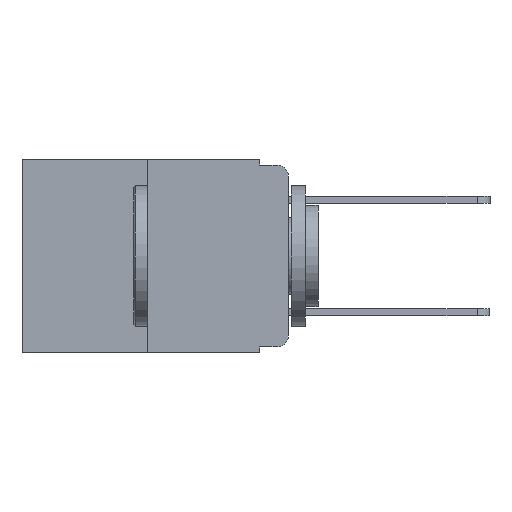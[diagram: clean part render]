
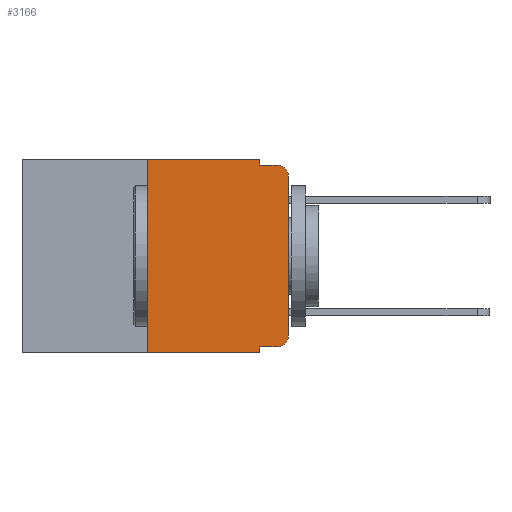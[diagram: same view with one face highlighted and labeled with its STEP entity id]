
A CAD part, left-side view. The second image highlights one B-rep face of the part: STEP entity #3166.
In plain terms, the highlighted planar face has unit normal (-1, 0, 0).
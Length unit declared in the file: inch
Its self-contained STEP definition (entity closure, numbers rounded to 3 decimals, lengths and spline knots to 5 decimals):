
#98 = CARTESIAN_POINT ( 'NONE',  ( 0., 0.25, 0. ) ) ;
#194 = CARTESIAN_POINT ( 'NONE',  ( 0., 0.02, -0.03 ) ) ;
#332 = LINE ( 'NONE', #822, #599 ) ;
#370 = VERTEX_POINT ( 'NONE', #8942 ) ;
#573 = EDGE_LOOP ( 'NONE', ( #9256, #2607, #1830, #5777, #4841, #9421, #8295, #3054, #5703, #5567 ) ) ;
#583 = CARTESIAN_POINT ( 'NONE',  ( 0., 0., -0.313 ) ) ;
#599 = VECTOR ( 'NONE', #7869, 39.37008 ) ;
#763 = CARTESIAN_POINT ( 'NONE',  ( 0., 0., -0.03 ) ) ;
#764 = AXIS2_PLACEMENT_3D ( 'NONE', #11268, #3282, #7106 ) ;
#777 = EDGE_CURVE ( 'NONE', #8177, #5289, #7945, .T. ) ;
#822 = CARTESIAN_POINT ( 'NONE',  ( 0., 0.473, -0.343 ) ) ;
#921 = VERTEX_POINT ( 'NONE', #9349 ) ;
#936 = DIRECTION ( 'NONE',  ( 0., 0., -1. ) ) ;
#1016 = PLANE ( 'NONE',  #6202 ) ;
#1062 = DIRECTION ( 'NONE',  ( 1., 0., 0. ) ) ;
#1086 = DIRECTION ( 'NONE',  ( 0., 0., -1. ) ) ;
#1391 = VERTEX_POINT ( 'NONE', #7061 ) ;
#1514 = DIRECTION ( 'NONE',  ( 0., -1., 0. ) ) ;
#1668 = EDGE_CURVE ( 'NONE', #5289, #6997, #3530, .T. ) ;
#1695 = EDGE_CURVE ( 'NONE', #2657, #9983, #5552, .T. ) ;
#1740 = VERTEX_POINT ( 'NONE', #7189 ) ;
#1830 = ORIENTED_EDGE ( 'NONE', *, *, #10908, .F. ) ;
#2138 = CARTESIAN_POINT ( 'NONE',  ( 0., 0.25, -0.343 ) ) ;
#2457 = LINE ( 'NONE', #3936, #9016 ) ;
#2587 = VECTOR ( 'NONE', #1514, 39.37008 ) ;
#2607 = ORIENTED_EDGE ( 'NONE', *, *, #9808, .T. ) ;
#2657 = VERTEX_POINT ( 'NONE', #2138 ) ;
#2955 = CARTESIAN_POINT ( 'NONE',  ( 0., 0.473, 0. ) ) ;
#3054 = ORIENTED_EDGE ( 'NONE', *, *, #4827, .F. ) ;
#3144 = VECTOR ( 'NONE', #8065, 39.37008 ) ;
#3166 = ADVANCED_FACE ( 'NONE', ( #9590 ), #1016, .F. ) ;
#3282 = DIRECTION ( 'NONE',  ( -1., 0., 0. ) ) ;
#3530 = LINE ( 'NONE', #10547, #8180 ) ;
#3936 = CARTESIAN_POINT ( 'NONE',  ( 0., 0.473, 0. ) ) ;
#4038 = DIRECTION ( 'NONE',  ( 0., -1., 0. ) ) ;
#4348 = CARTESIAN_POINT ( 'NONE',  ( 0., 0.25, 0. ) ) ;
#4811 = DIRECTION ( 'NONE',  ( 0., -1., 0. ) ) ;
#4827 = EDGE_CURVE ( 'NONE', #921, #11189, #8529, .T. ) ;
#4841 = ORIENTED_EDGE ( 'NONE', *, *, #8213, .F. ) ;
#5021 = DIRECTION ( 'NONE',  ( 0., 0., 1. ) ) ;
#5023 = LINE ( 'NONE', #6848, #2587 ) ;
#5289 = VERTEX_POINT ( 'NONE', #583 ) ;
#5552 = LINE ( 'NONE', #4348, #7435 ) ;
#5567 = ORIENTED_EDGE ( 'NONE', *, *, #777, .T. ) ;
#5686 = CARTESIAN_POINT ( 'NONE',  ( 0., 0.051, 0. ) ) ;
#5697 = CARTESIAN_POINT ( 'NONE',  ( 0., 0.051, -0.01 ) ) ;
#5703 = ORIENTED_EDGE ( 'NONE', *, *, #9442, .T. ) ;
#5777 = ORIENTED_EDGE ( 'NONE', *, *, #5788, .F. ) ;
#5788 = EDGE_CURVE ( 'NONE', #1391, #1740, #7616, .T. ) ;
#6202 = AXIS2_PLACEMENT_3D ( 'NONE', #2955, #1062, #936 ) ;
#6388 = VECTOR ( 'NONE', #8837, 39.37008 ) ;
#6494 = DIRECTION ( 'NONE',  ( -1., 0., 0. ) ) ;
#6788 = CIRCLE ( 'NONE', #8379, 0.02 ) ;
#6848 = CARTESIAN_POINT ( 'NONE',  ( 0., 0.051, -0.333 ) ) ;
#6997 = VERTEX_POINT ( 'NONE', #763 ) ;
#7028 = VECTOR ( 'NONE', #4038, 39.37008 ) ;
#7061 = CARTESIAN_POINT ( 'NONE',  ( 0., 0.051, 0. ) ) ;
#7106 = DIRECTION ( 'NONE',  ( 0., 0., -1. ) ) ;
#7189 = CARTESIAN_POINT ( 'NONE',  ( 0., 0.051, -0.01 ) ) ;
#7435 = VECTOR ( 'NONE', #5021, 39.37008 ) ;
#7616 = LINE ( 'NONE', #5686, #3144 ) ;
#7869 = DIRECTION ( 'NONE',  ( 0., -1., 0. ) ) ;
#7945 = CIRCLE ( 'NONE', #764, 0.02 ) ;
#7971 = CARTESIAN_POINT ( 'NONE',  ( 0., 0.051, 0. ) ) ;
#8065 = DIRECTION ( 'NONE',  ( 0., 0., -1. ) ) ;
#8177 = VERTEX_POINT ( 'NONE', #10521 ) ;
#8180 = VECTOR ( 'NONE', #10480, 39.37008 ) ;
#8213 = EDGE_CURVE ( 'NONE', #9983, #1391, #2457, .T. ) ;
#8295 = ORIENTED_EDGE ( 'NONE', *, *, #10646, .T. ) ;
#8379 = AXIS2_PLACEMENT_3D ( 'NONE', #194, #6494, #1086 ) ;
#8529 = LINE ( 'NONE', #7971, #6388 ) ;
#8837 = DIRECTION ( 'NONE',  ( 0., 0., -1. ) ) ;
#8942 = CARTESIAN_POINT ( 'NONE',  ( 0., 0.02, -0.01 ) ) ;
#9016 = VECTOR ( 'NONE', #4811, 39.37008 ) ;
#9246 = LINE ( 'NONE', #5697, #7028 ) ;
#9256 = ORIENTED_EDGE ( 'NONE', *, *, #1668, .T. ) ;
#9291 = CARTESIAN_POINT ( 'NONE',  ( 0., 0.051, -0.343 ) ) ;
#9349 = CARTESIAN_POINT ( 'NONE',  ( 0., 0.051, -0.333 ) ) ;
#9421 = ORIENTED_EDGE ( 'NONE', *, *, #1695, .F. ) ;
#9442 = EDGE_CURVE ( 'NONE', #921, #8177, #5023, .T. ) ;
#9590 = FACE_OUTER_BOUND ( 'NONE', #573, .T. ) ;
#9808 = EDGE_CURVE ( 'NONE', #6997, #370, #6788, .T. ) ;
#9983 = VERTEX_POINT ( 'NONE', #98 ) ;
#10480 = DIRECTION ( 'NONE',  ( 0., 0., 1. ) ) ;
#10521 = CARTESIAN_POINT ( 'NONE',  ( 0., 0.02, -0.333 ) ) ;
#10547 = CARTESIAN_POINT ( 'NONE',  ( 0., 0., 0. ) ) ;
#10646 = EDGE_CURVE ( 'NONE', #2657, #11189, #332, .T. ) ;
#10908 = EDGE_CURVE ( 'NONE', #1740, #370, #9246, .T. ) ;
#11189 = VERTEX_POINT ( 'NONE', #9291 ) ;
#11268 = CARTESIAN_POINT ( 'NONE',  ( 0., 0.02, -0.313 ) ) ;
